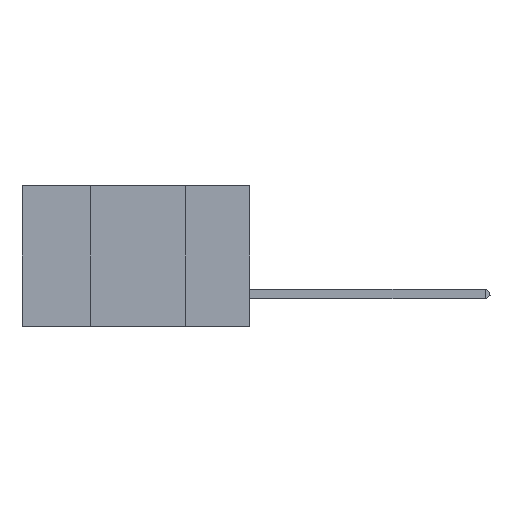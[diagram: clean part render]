
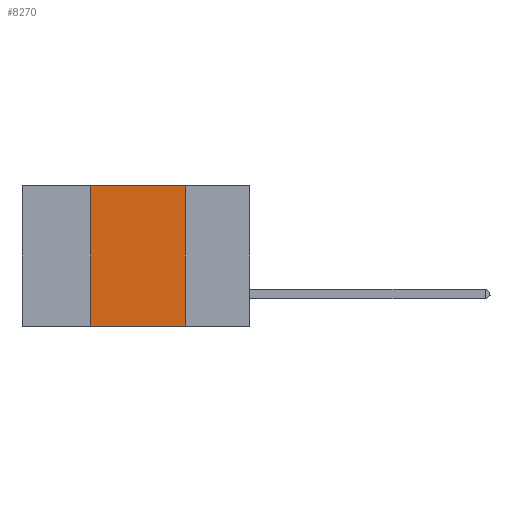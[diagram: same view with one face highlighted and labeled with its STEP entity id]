
A CAD part, left-side view. The second image highlights one B-rep face of the part: STEP entity #8270.
In plain terms, the highlighted planar face has unit normal (-1, 0, 0).
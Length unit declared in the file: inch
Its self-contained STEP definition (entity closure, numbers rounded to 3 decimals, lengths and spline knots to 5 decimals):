
#2069 = VERTEX_POINT ( 'NONE', #11229 ) ;
#2336 = DIRECTION ( 'NONE',  ( 0., 0., 1. ) ) ;
#2751 = VECTOR ( 'NONE', #9716, 39.37008 ) ;
#4042 = LINE ( 'NONE', #28709, #2751 ) ;
#4132 = LINE ( 'NONE', #7258, #19427 ) ;
#4366 = LINE ( 'NONE', #32226, #5289 ) ;
#4372 = DIRECTION ( 'NONE',  ( 0., 0., -1. ) ) ;
#5289 = VECTOR ( 'NONE', #35010, 39.37008 ) ;
#6479 = VECTOR ( 'NONE', #2336, 39.37008 ) ;
#7258 = CARTESIAN_POINT ( 'NONE',  ( 0., 0.6, 0. ) ) ;
#8216 = CARTESIAN_POINT ( 'NONE',  ( 0., 0.42, 0. ) ) ;
#8270 = ADVANCED_FACE ( 'NONE', ( #13302 ), #26632, .F. ) ;
#8497 = VERTEX_POINT ( 'NONE', #24458 ) ;
#9716 = DIRECTION ( 'NONE',  ( 0., -1., 0. ) ) ;
#9857 = DIRECTION ( 'NONE',  ( 1., 0., 0. ) ) ;
#9901 = VERTEX_POINT ( 'NONE', #32867 ) ;
#11229 = CARTESIAN_POINT ( 'NONE',  ( 0., 0.17, -0.37 ) ) ;
#12333 = EDGE_CURVE ( 'NONE', #8497, #32454, #4132, .T. ) ;
#12820 = DIRECTION ( 'NONE',  ( 0., -1., 0. ) ) ;
#13302 = FACE_OUTER_BOUND ( 'NONE', #16133, .T. ) ;
#13908 = LINE ( 'NONE', #8216, #6479 ) ;
#16133 = EDGE_LOOP ( 'NONE', ( #34721, #29071, #22383, #22092 ) ) ;
#18036 = AXIS2_PLACEMENT_3D ( 'NONE', #18133, #9857, #4372 ) ;
#18133 = CARTESIAN_POINT ( 'NONE',  ( 0., 0.6, 0. ) ) ;
#19427 = VECTOR ( 'NONE', #12820, 39.37008 ) ;
#22092 = ORIENTED_EDGE ( 'NONE', *, *, #27991, .T. ) ;
#22383 = ORIENTED_EDGE ( 'NONE', *, *, #33860, .F. ) ;
#24458 = CARTESIAN_POINT ( 'NONE',  ( 0., 0.42, 0. ) ) ;
#26632 = PLANE ( 'NONE',  #18036 ) ;
#27991 = EDGE_CURVE ( 'NONE', #9901, #2069, #4042, .T. ) ;
#28709 = CARTESIAN_POINT ( 'NONE',  ( 0., 0.6, -0.37 ) ) ;
#29071 = ORIENTED_EDGE ( 'NONE', *, *, #12333, .F. ) ;
#29941 = EDGE_CURVE ( 'NONE', #32454, #2069, #4366, .T. ) ;
#32226 = CARTESIAN_POINT ( 'NONE',  ( 0., 0.17, 0. ) ) ;
#32454 = VERTEX_POINT ( 'NONE', #33255 ) ;
#32867 = CARTESIAN_POINT ( 'NONE',  ( 0., 0.42, -0.37 ) ) ;
#33255 = CARTESIAN_POINT ( 'NONE',  ( 0., 0.17, 0. ) ) ;
#33860 = EDGE_CURVE ( 'NONE', #9901, #8497, #13908, .T. ) ;
#34721 = ORIENTED_EDGE ( 'NONE', *, *, #29941, .F. ) ;
#35010 = DIRECTION ( 'NONE',  ( 0., 0., -1. ) ) ;
